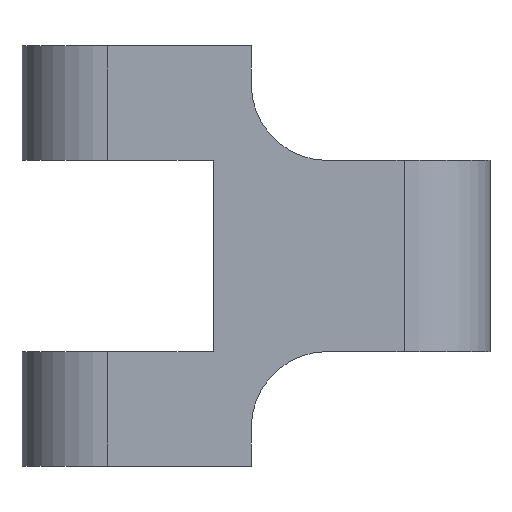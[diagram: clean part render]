
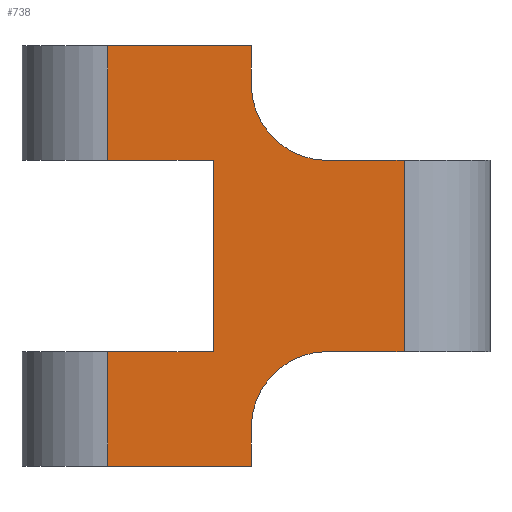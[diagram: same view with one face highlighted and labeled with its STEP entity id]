
A CAD part, front view. The second image highlights one B-rep face of the part: STEP entity #738.
In plain terms, the highlighted planar face has unit normal (0, -1, 0).
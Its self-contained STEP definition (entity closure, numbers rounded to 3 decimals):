
#4 = VECTOR ( 'NONE', #340, 1000. ) ;
#25 = EDGE_CURVE ( 'NONE', #693, #33, #202, .T. ) ;
#28 = EDGE_CURVE ( 'NONE', #353, #693, #626, .T. ) ;
#32 = LINE ( 'NONE', #646, #80 ) ;
#33 = VERTEX_POINT ( 'NONE', #277 ) ;
#39 = AXIS2_PLACEMENT_3D ( 'NONE', #772, #239, #243 ) ;
#42 = ORIENTED_EDGE ( 'NONE', *, *, #25, .T. ) ;
#44 = CARTESIAN_POINT ( 'NONE',  ( 11.5, -4.5, 14. ) ) ;
#45 = DIRECTION ( 'NONE',  ( 1., 0., 0. ) ) ;
#49 = DIRECTION ( 'NONE',  ( 0., 0., 1. ) ) ;
#52 = AXIS2_PLACEMENT_3D ( 'NONE', #44, #364, #420 ) ;
#63 = EDGE_CURVE ( 'NONE', #485, #721, #269, .T. ) ;
#67 = CARTESIAN_POINT ( 'NONE',  ( 0., -4.5, -6. ) ) ;
#68 = VECTOR ( 'NONE', #573, 1000. ) ;
#69 = CARTESIAN_POINT ( 'NONE',  ( 7.5, -4.5, 16. ) ) ;
#77 = ORIENTED_EDGE ( 'NONE', *, *, #123, .F. ) ;
#79 = DIRECTION ( 'NONE',  ( 0., 0., -1. ) ) ;
#80 = VECTOR ( 'NONE', #45, 1000. ) ;
#82 = EDGE_CURVE ( 'NONE', #331, #725, #680, .T. ) ;
#84 = CARTESIAN_POINT ( 'NONE',  ( 0., -4.5, -6. ) ) ;
#90 = VERTEX_POINT ( 'NONE', #579 ) ;
#96 = VERTEX_POINT ( 'NONE', #766 ) ;
#98 = ORIENTED_EDGE ( 'NONE', *, *, #765, .T. ) ;
#99 = CARTESIAN_POINT ( 'NONE',  ( 11.5, -4.5, 10. ) ) ;
#103 = CARTESIAN_POINT ( 'NONE',  ( 11.5, -4.5, -4. ) ) ;
#109 = ORIENTED_EDGE ( 'NONE', *, *, #82, .T. ) ;
#110 = EDGE_CURVE ( 'NONE', #718, #485, #32, .T. ) ;
#117 = CIRCLE ( 'NONE', #396, 4. ) ;
#123 = EDGE_CURVE ( 'NONE', #759, #96, #232, .T. ) ;
#135 = CARTESIAN_POINT ( 'NONE',  ( 5.5, -4.5, 0. ) ) ;
#148 = VECTOR ( 'NONE', #557, 1000. ) ;
#159 = VECTOR ( 'NONE', #375, 1000. ) ;
#163 = CARTESIAN_POINT ( 'NONE',  ( 15.5, -4.5, 10. ) ) ;
#175 = EDGE_CURVE ( 'NONE', #718, #714, #752, .T. ) ;
#177 = EDGE_CURVE ( 'NONE', #90, #725, #638, .T. ) ;
#197 = ORIENTED_EDGE ( 'NONE', *, *, #454, .T. ) ;
#202 = LINE ( 'NONE', #442, #148 ) ;
#205 = EDGE_CURVE ( 'NONE', #353, #759, #541, .T. ) ;
#216 = ORIENTED_EDGE ( 'NONE', *, *, #678, .T. ) ;
#232 = LINE ( 'NONE', #391, #4 ) ;
#239 = DIRECTION ( 'NONE',  ( 0., -1., 0. ) ) ;
#243 = DIRECTION ( 'NONE',  ( 1., 0., 0. ) ) ;
#254 = LINE ( 'NONE', #555, #159 ) ;
#265 = LINE ( 'NONE', #553, #275 ) ;
#269 = LINE ( 'NONE', #69, #387 ) ;
#270 = EDGE_CURVE ( 'NONE', #510, #90, #352, .T. ) ;
#275 = VECTOR ( 'NONE', #79, 1000. ) ;
#277 = CARTESIAN_POINT ( 'NONE',  ( 7.5, -4.5, -4. ) ) ;
#297 = DIRECTION ( 'NONE',  ( 1., 0., 0. ) ) ;
#300 = ORIENTED_EDGE ( 'NONE', *, *, #270, .F. ) ;
#322 = DIRECTION ( 'NONE',  ( 1., 0., 0. ) ) ;
#325 = CIRCLE ( 'NONE', #52, 4. ) ;
#331 = VERTEX_POINT ( 'NONE', #615 ) ;
#340 = DIRECTION ( 'NONE',  ( 1., 0., 0. ) ) ;
#352 = LINE ( 'NONE', #602, #467 ) ;
#353 = VERTEX_POINT ( 'NONE', #67 ) ;
#355 = DIRECTION ( 'NONE',  ( 0., 1., 0. ) ) ;
#364 = DIRECTION ( 'NONE',  ( 0., 1., 0. ) ) ;
#370 = CARTESIAN_POINT ( 'NONE',  ( 0., -4.5, 0. ) ) ;
#373 = ORIENTED_EDGE ( 'NONE', *, *, #205, .F. ) ;
#375 = DIRECTION ( 'NONE',  ( 1., 0., 0. ) ) ;
#387 = VECTOR ( 'NONE', #438, 1000. ) ;
#391 = CARTESIAN_POINT ( 'NONE',  ( 0., -4.5, 0. ) ) ;
#396 = AXIS2_PLACEMENT_3D ( 'NONE', #103, #355, #297 ) ;
#401 = DIRECTION ( 'NONE',  ( 0., 0., -1. ) ) ;
#402 = VERTEX_POINT ( 'NONE', #444 ) ;
#406 = ORIENTED_EDGE ( 'NONE', *, *, #177, .F. ) ;
#408 = CARTESIAN_POINT ( 'NONE',  ( 7.5, -4.5, 14. ) ) ;
#420 = DIRECTION ( 'NONE',  ( 1., 0., 0. ) ) ;
#429 = CARTESIAN_POINT ( 'NONE',  ( 0., -4.5, -6. ) ) ;
#438 = DIRECTION ( 'NONE',  ( 0., 0., -1. ) ) ;
#442 = CARTESIAN_POINT ( 'NONE',  ( 7.5, -4.5, -6. ) ) ;
#444 = CARTESIAN_POINT ( 'NONE',  ( 5.5, -4.5, 10. ) ) ;
#447 = CARTESIAN_POINT ( 'NONE',  ( 7.5, -4.5, 16. ) ) ;
#454 = EDGE_CURVE ( 'NONE', #402, #96, #265, .T. ) ;
#467 = VECTOR ( 'NONE', #669, 1000. ) ;
#470 = CARTESIAN_POINT ( 'NONE',  ( 0., -4.5, 16. ) ) ;
#485 = VERTEX_POINT ( 'NONE', #447 ) ;
#510 = VERTEX_POINT ( 'NONE', #99 ) ;
#517 = ORIENTED_EDGE ( 'NONE', *, *, #63, .F. ) ;
#518 = VECTOR ( 'NONE', #401, 1000. ) ;
#535 = PLANE ( 'NONE',  #39 ) ;
#541 = LINE ( 'NONE', #429, #749 ) ;
#553 = CARTESIAN_POINT ( 'NONE',  ( 5.5, -4.5, 10. ) ) ;
#554 = VECTOR ( 'NONE', #704, 1000. ) ;
#555 = CARTESIAN_POINT ( 'NONE',  ( 0., -4.5, 10. ) ) ;
#557 = DIRECTION ( 'NONE',  ( 0., 0., 1. ) ) ;
#570 = ORIENTED_EDGE ( 'NONE', *, *, #683, .T. ) ;
#573 = DIRECTION ( 'NONE',  ( 1., 0., 0. ) ) ;
#576 = ORIENTED_EDGE ( 'NONE', *, *, #110, .F. ) ;
#579 = CARTESIAN_POINT ( 'NONE',  ( 15.5, -4.5, 10. ) ) ;
#602 = CARTESIAN_POINT ( 'NONE',  ( 5.5, -4.5, 10. ) ) ;
#615 = CARTESIAN_POINT ( 'NONE',  ( 11.5, -4.5, 0. ) ) ;
#626 = LINE ( 'NONE', #84, #68 ) ;
#638 = LINE ( 'NONE', #163, #518 ) ;
#646 = CARTESIAN_POINT ( 'NONE',  ( 0., -4.5, 16. ) ) ;
#652 = ORIENTED_EDGE ( 'NONE', *, *, #28, .T. ) ;
#655 = CARTESIAN_POINT ( 'NONE',  ( 15.5, -4.5, 0. ) ) ;
#656 = VECTOR ( 'NONE', #322, 1000. ) ;
#659 = FACE_OUTER_BOUND ( 'NONE', #667, .T. ) ;
#663 = CARTESIAN_POINT ( 'NONE',  ( 7.5, -4.5, -6. ) ) ;
#667 = EDGE_LOOP ( 'NONE', ( #77, #373, #652, #42, #216, #109, #406, #300, #570, #517, #576, #676, #98, #197 ) ) ;
#669 = DIRECTION ( 'NONE',  ( 1., 0., 0. ) ) ;
#676 = ORIENTED_EDGE ( 'NONE', *, *, #175, .T. ) ;
#678 = EDGE_CURVE ( 'NONE', #33, #331, #117, .T. ) ;
#680 = LINE ( 'NONE', #135, #656 ) ;
#683 = EDGE_CURVE ( 'NONE', #510, #721, #325, .T. ) ;
#693 = VERTEX_POINT ( 'NONE', #663 ) ;
#704 = DIRECTION ( 'NONE',  ( 0., 0., -1. ) ) ;
#714 = VERTEX_POINT ( 'NONE', #719 ) ;
#718 = VERTEX_POINT ( 'NONE', #783 ) ;
#719 = CARTESIAN_POINT ( 'NONE',  ( 0., -4.5, 10. ) ) ;
#721 = VERTEX_POINT ( 'NONE', #408 ) ;
#725 = VERTEX_POINT ( 'NONE', #655 ) ;
#738 = ADVANCED_FACE ( 'NONE', ( #659 ), #535, .T. ) ;
#749 = VECTOR ( 'NONE', #49, 1000. ) ;
#752 = LINE ( 'NONE', #470, #554 ) ;
#759 = VERTEX_POINT ( 'NONE', #370 ) ;
#765 = EDGE_CURVE ( 'NONE', #714, #402, #254, .T. ) ;
#766 = CARTESIAN_POINT ( 'NONE',  ( 5.5, -4.5, 0. ) ) ;
#772 = CARTESIAN_POINT ( 'NONE',  ( 0., -4.5, -6. ) ) ;
#783 = CARTESIAN_POINT ( 'NONE',  ( 0., -4.5, 16. ) ) ;
